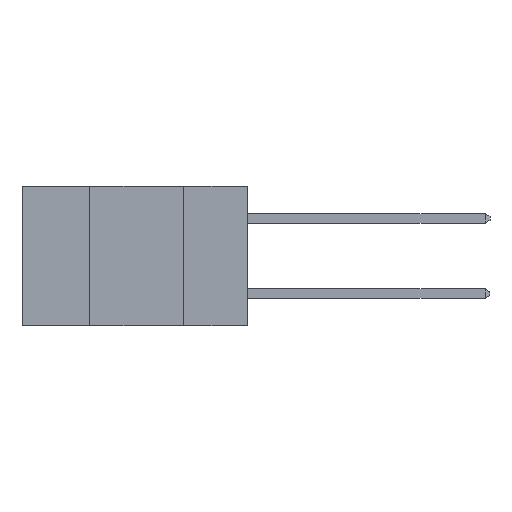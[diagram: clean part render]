
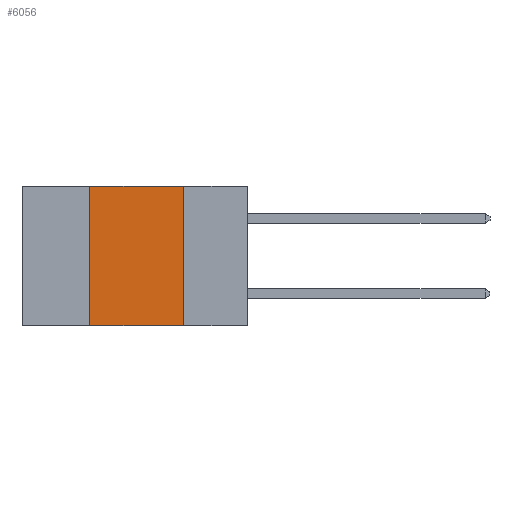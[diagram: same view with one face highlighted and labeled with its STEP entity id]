
A CAD part, left-side view. The second image highlights one B-rep face of the part: STEP entity #6056.
In plain terms, the highlighted planar face has unit normal (-1, 0, 0).
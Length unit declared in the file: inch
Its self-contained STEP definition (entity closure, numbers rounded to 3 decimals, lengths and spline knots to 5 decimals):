
#6 = DIRECTION ( 'NONE',  ( 0., -1., 0. ) ) ;
#114 = ORIENTED_EDGE ( 'NONE', *, *, #772, .T. ) ;
#191 = DIRECTION ( 'NONE',  ( 0., -1., 0. ) ) ;
#324 = EDGE_CURVE ( 'NONE', #5438, #9625, #10105, .T. ) ;
#508 = DIRECTION ( 'NONE',  ( 0., 0., -1. ) ) ;
#685 = EDGE_CURVE ( 'NONE', #8930, #5386, #8832, .T. ) ;
#772 = EDGE_CURVE ( 'NONE', #8930, #9625, #2139, .T. ) ;
#1210 = FACE_OUTER_BOUND ( 'NONE', #5590, .T. ) ;
#1894 = VECTOR ( 'NONE', #191, 39.37008 ) ;
#1902 = VECTOR ( 'NONE', #4235, 39.37008 ) ;
#2139 = LINE ( 'NONE', #8206, #1894 ) ;
#2344 = CARTESIAN_POINT ( 'NONE',  ( 0., 0.42, 0. ) ) ;
#2625 = VECTOR ( 'NONE', #6, 39.37008 ) ;
#2646 = VECTOR ( 'NONE', #7297, 39.37008 ) ;
#2852 = CARTESIAN_POINT ( 'NONE',  ( 0., 0.6, 0. ) ) ;
#3452 = AXIS2_PLACEMENT_3D ( 'NONE', #2852, #4613, #508 ) ;
#3534 = CARTESIAN_POINT ( 'NONE',  ( 0., 0.42, -0.37 ) ) ;
#4208 = PLANE ( 'NONE',  #3452 ) ;
#4235 = DIRECTION ( 'NONE',  ( 0., 0., -1. ) ) ;
#4613 = DIRECTION ( 'NONE',  ( 1., 0., 0. ) ) ;
#5386 = VERTEX_POINT ( 'NONE', #8048 ) ;
#5438 = VERTEX_POINT ( 'NONE', #9967 ) ;
#5590 = EDGE_LOOP ( 'NONE', ( #9408, #9458, #9582, #114 ) ) ;
#5914 = CARTESIAN_POINT ( 'NONE',  ( 0., 0.17, -0.37 ) ) ;
#6056 = ADVANCED_FACE ( 'NONE', ( #1210 ), #4208, .F. ) ;
#6440 = CARTESIAN_POINT ( 'NONE',  ( 0., 0.6, 0. ) ) ;
#6933 = CARTESIAN_POINT ( 'NONE',  ( 0., 0.17, 0. ) ) ;
#7297 = DIRECTION ( 'NONE',  ( 0., 0., 1. ) ) ;
#8048 = CARTESIAN_POINT ( 'NONE',  ( 0., 0.42, 0. ) ) ;
#8133 = EDGE_CURVE ( 'NONE', #5386, #5438, #9050, .T. ) ;
#8206 = CARTESIAN_POINT ( 'NONE',  ( 0., 0.6, -0.37 ) ) ;
#8832 = LINE ( 'NONE', #2344, #2646 ) ;
#8930 = VERTEX_POINT ( 'NONE', #3534 ) ;
#9050 = LINE ( 'NONE', #6440, #2625 ) ;
#9408 = ORIENTED_EDGE ( 'NONE', *, *, #324, .F. ) ;
#9458 = ORIENTED_EDGE ( 'NONE', *, *, #8133, .F. ) ;
#9582 = ORIENTED_EDGE ( 'NONE', *, *, #685, .F. ) ;
#9625 = VERTEX_POINT ( 'NONE', #5914 ) ;
#9967 = CARTESIAN_POINT ( 'NONE',  ( 0., 0.17, 0. ) ) ;
#10105 = LINE ( 'NONE', #6933, #1902 ) ;
